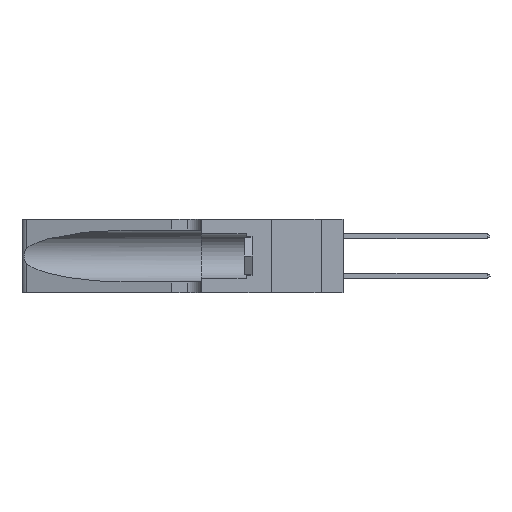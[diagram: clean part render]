
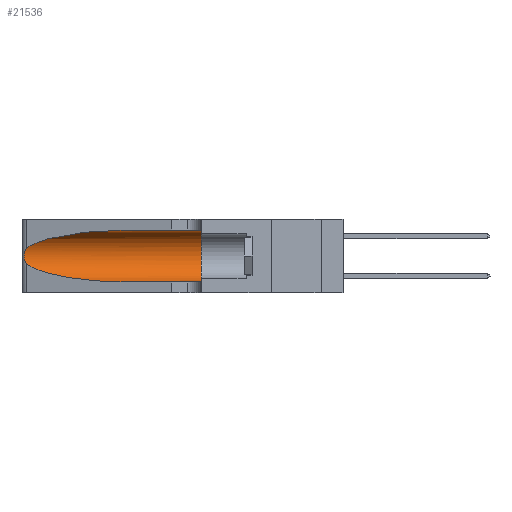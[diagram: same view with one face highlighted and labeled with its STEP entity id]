
A CAD part, left-side view. The second image highlights one B-rep face of the part: STEP entity #21536.
In plain terms, the highlighted cylindrical face has radius 3.308 mm (diameter 6.617 mm), a partial arc.
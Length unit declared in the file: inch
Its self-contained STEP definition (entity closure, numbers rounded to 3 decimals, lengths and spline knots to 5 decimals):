
#651 = CARTESIAN_POINT ( 'NONE',  ( 0.1305, 1.61858, 0.185 ) ) ;
#926 = CARTESIAN_POINT ( 'NONE',  ( 0.1305, 0.72297, 0.05475 ) ) ;
#1097 = AXIS2_PLACEMENT_3D ( 'NONE', #651, #26157, #14395 ) ;
#1591 =( BOUNDED_CURVE ( )  B_SPLINE_CURVE ( 3, ( #11255, #15865, #15484, #22701 ),
 .UNSPECIFIED., .F., .T. ) 
 B_SPLINE_CURVE_WITH_KNOTS ( ( 4, 4 ),
 ( 1.5708, 2.84003 ),
 .UNSPECIFIED. ) 
 CURVE ( )  GEOMETRIC_REPRESENTATION_ITEM ( )  RATIONAL_B_SPLINE_CURVE ( ( 1., 0.87, 0.87, 1. ) ) 
 REPRESENTATION_ITEM ( '' )  );
#1612 = CARTESIAN_POINT ( 'NONE',  ( 0.26018, 1.23835, 0.19895 ) ) ;
#1691 = CARTESIAN_POINT ( 'NONE',  ( 0.1305, 1.61858, 0.31525 ) ) ;
#2998 = EDGE_CURVE ( 'NONE', #5048, #9041, #26496, .T. ) ;
#3242 = CARTESIAN_POINT ( 'NONE',  ( 0.25487, 1.22718, 0.22369 ) ) ;
#3589 = DIRECTION ( 'NONE',  ( 0., 0., 1. ) ) ;
#4585 = VECTOR ( 'NONE', #28218, 39.37008 ) ;
#5018 = FACE_OUTER_BOUND ( 'NONE', #19866, .T. ) ;
#5048 = VERTEX_POINT ( 'NONE', #16125 ) ;
#5876 = CARTESIAN_POINT ( 'NONE',  ( 0.26075, 1.23896, 0.19203 ) ) ;
#6127 = CARTESIAN_POINT ( 'NONE',  ( 0.2373, 1.15595, 0.08982 ) ) ;
#6397 = LINE ( 'NONE', #23662, #4585 ) ;
#8060 = CARTESIAN_POINT ( 'NONE',  ( 0.25487, 1.22718, 0.14631 ) ) ;
#8394 = CARTESIAN_POINT ( 'NONE',  ( 0.25487, 1.22718, 0.22369 ) ) ;
#9036 = CIRCLE ( 'NONE', #16007, 0.13025 ) ;
#9041 = VERTEX_POINT ( 'NONE', #926 ) ;
#9164 = ORIENTED_EDGE ( 'NONE', *, *, #2998, .T. ) ;
#10563 = EDGE_CURVE ( 'NONE', #21676, #19929, #9036, .T. ) ;
#10733 = CARTESIAN_POINT ( 'NONE',  ( 0.25639, 1.23184, 0.21858 ) ) ;
#11255 = CARTESIAN_POINT ( 'NONE',  ( 0.1305, 0.72297, 0.31525 ) ) ;
#11822 = VECTOR ( 'NONE', #23195, 39.37008 ) ;
#12824 = CARTESIAN_POINT ( 'NONE',  ( 0.25555, 1.22993, 0.14849 ) ) ;
#12857 = CARTESIAN_POINT ( 'NONE',  ( 0.1305, 0.72297, 0.31525 ) ) ;
#13016 = CARTESIAN_POINT ( 'NONE',  ( 0.26075, 1.23896, 0.178 ) ) ;
#13090 = CARTESIAN_POINT ( 'NONE',  ( 0.1305, 0.35, 0.185 ) ) ;
#14395 = DIRECTION ( 'NONE',  ( 0., 0., -1. ) ) ;
#14725 = LINE ( 'NONE', #1691, #11822 ) ;
#14770 = ORIENTED_EDGE ( 'NONE', *, *, #10563, .F. ) ;
#15363 = CARTESIAN_POINT ( 'NONE',  ( 0.25487, 1.22718, 0.14631 ) ) ;
#15484 = CARTESIAN_POINT ( 'NONE',  ( 0.2373, 1.15595, 0.28018 ) ) ;
#15865 = CARTESIAN_POINT ( 'NONE',  ( 0.18966, 0.96281, 0.31525 ) ) ;
#16007 = AXIS2_PLACEMENT_3D ( 'NONE', #13090, #28910, #3589 ) ;
#16099 = EDGE_CURVE ( 'NONE', #23589, #21676, #14725, .T. ) ;
#16125 = CARTESIAN_POINT ( 'NONE',  ( 0.25487, 1.22718, 0.14631 ) ) ;
#16487 = ORIENTED_EDGE ( 'NONE', *, *, #24399, .T. ) ;
#17452 = CARTESIAN_POINT ( 'NONE',  ( 0.18966, 0.96281, 0.05475 ) ) ;
#18974 = VERTEX_POINT ( 'NONE', #3242 ) ;
#19684 = CARTESIAN_POINT ( 'NONE',  ( 0.25854, 1.2359, 0.20912 ) ) ;
#19745 = CARTESIAN_POINT ( 'NONE',  ( 0.1305, 0.35, 0.31525 ) ) ;
#19866 = EDGE_LOOP ( 'NONE', ( #27472, #16487, #9164, #23858, #14770, #20990 ) ) ;
#19929 = VERTEX_POINT ( 'NONE', #20215 ) ;
#20069 = CARTESIAN_POINT ( 'NONE',  ( 0.25639, 1.23186, 0.15144 ) ) ;
#20215 = CARTESIAN_POINT ( 'NONE',  ( 0.1305, 0.35, 0.05475 ) ) ;
#20990 = ORIENTED_EDGE ( 'NONE', *, *, #16099, .F. ) ;
#21536 = ADVANCED_FACE ( 'NONE', ( #5018 ), #22320, .F. ) ;
#21676 = VERTEX_POINT ( 'NONE', #19745 ) ;
#22078 = CARTESIAN_POINT ( 'NONE',  ( 0.25856, 1.23593, 0.16098 ) ) ;
#22320 = CYLINDRICAL_SURFACE ( 'NONE', #1097, 0.13025 ) ;
#22701 = CARTESIAN_POINT ( 'NONE',  ( 0.25487, 1.22718, 0.22369 ) ) ;
#23010 = B_SPLINE_CURVE_WITH_KNOTS ( 'NONE', 3,
 ( #8394, #27005, #10733, #26911, #19684, #1612, #5876, #13016, #29142, #22078, #26607, #20069, #12824, #15363 ),
 .UNSPECIFIED., .F., .F.,
 ( 4, 2, 2, 2, 2, 2, 4 ),
 ( 0., 0.00027, 0.00053, 0.00107, 0.0016, 0.00187, 0.00214 ),
 .UNSPECIFIED. ) ;
#23195 = DIRECTION ( 'NONE',  ( 0., -1., 0. ) ) ;
#23589 = VERTEX_POINT ( 'NONE', #12857 ) ;
#23662 = CARTESIAN_POINT ( 'NONE',  ( 0.1305, 1.61858, 0.05475 ) ) ;
#23737 = EDGE_CURVE ( 'NONE', #23589, #18974, #1591, .T. ) ;
#23858 = ORIENTED_EDGE ( 'NONE', *, *, #28325, .T. ) ;
#24170 = CARTESIAN_POINT ( 'NONE',  ( 0.1305, 0.72297, 0.05475 ) ) ;
#24399 = EDGE_CURVE ( 'NONE', #18974, #5048, #23010, .T. ) ;
#26157 = DIRECTION ( 'NONE',  ( 0., -1., 0. ) ) ;
#26496 =( BOUNDED_CURVE ( )  B_SPLINE_CURVE ( 3, ( #8060, #6127, #17452, #24170 ),
 .UNSPECIFIED., .F., .T. ) 
 B_SPLINE_CURVE_WITH_KNOTS ( ( 4, 4 ),
 ( 3.44316, 4.71239 ),
 .UNSPECIFIED. ) 
 CURVE ( )  GEOMETRIC_REPRESENTATION_ITEM ( )  RATIONAL_B_SPLINE_CURVE ( ( 1., 0.87, 0.87, 1. ) ) 
 REPRESENTATION_ITEM ( '' )  );
#26607 = CARTESIAN_POINT ( 'NONE',  ( 0.25789, 1.23486, 0.15765 ) ) ;
#26911 = CARTESIAN_POINT ( 'NONE',  ( 0.25787, 1.23484, 0.2124 ) ) ;
#27005 = CARTESIAN_POINT ( 'NONE',  ( 0.25555, 1.22994, 0.2215 ) ) ;
#27472 = ORIENTED_EDGE ( 'NONE', *, *, #23737, .T. ) ;
#28218 = DIRECTION ( 'NONE',  ( 0., -1., 0. ) ) ;
#28325 = EDGE_CURVE ( 'NONE', #9041, #19929, #6397, .T. ) ;
#28910 = DIRECTION ( 'NONE',  ( 0., 1., 0. ) ) ;
#29142 = CARTESIAN_POINT ( 'NONE',  ( 0.26017, 1.23833, 0.17102 ) ) ;
